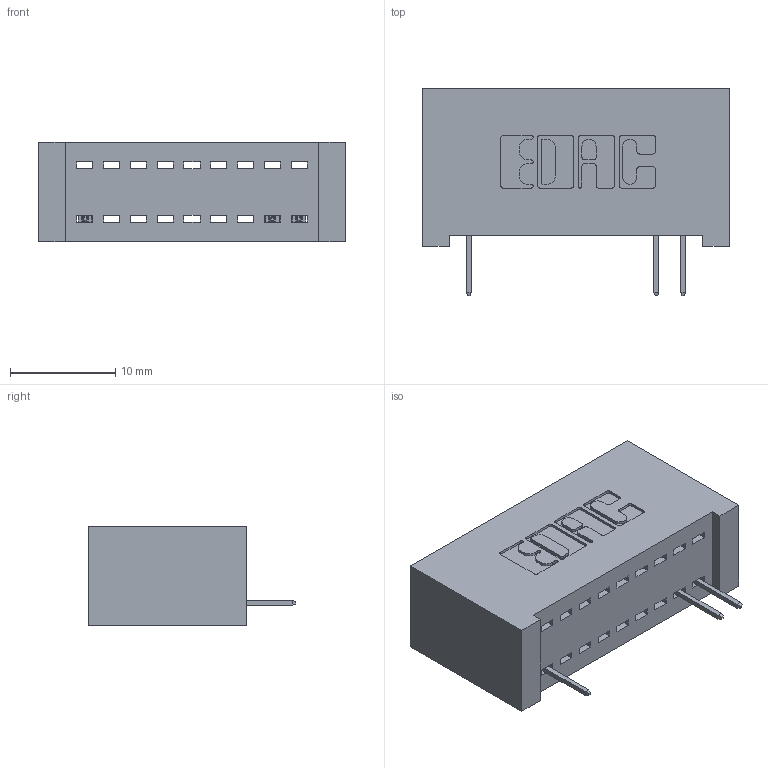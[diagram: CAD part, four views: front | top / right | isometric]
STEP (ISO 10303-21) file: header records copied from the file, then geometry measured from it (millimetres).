
FILE_DESCRIPTION (( 'STEP AP203' ), '1' );
FILE_NAME ('392-009-524-101.STEP', '2018-08-14T19:42:58', ( '' ), ( '' ), 'SwSTEP 2.0', 'SolidWorks 2016', '' );
FILE_SCHEMA (( 'CONFIG_CONTROL_DESIGN' ));
Length unit declared in the file: inch
Products named in the file (3): 345-292-001_345-293-124; 392-009-524-101; 342 Part_Lugless
Assembly tree (4 placements, depth 2):
  392-009-524-101
    342 Part_Lugless
    345-292-001_345-293-124  x3
Bounding box: 29.11 x 19.69 x 9.4 mm (x, y, z)
Volume: 2759.2 mm3; surface area: 3366.5 mm2
Topology: 4 solids, 4 shells, 360 faces, 1067 edges, 698 vertices
Faces by surface type: plane 278, cylinder 82
Entity records: 9243 total; most frequent: CARTESIAN_POINT 1631, ORIENTED_EDGE 1582, DIRECTION 1429, EDGE_CURVE 791, VECTOR 675, LINE 675, VERTEX_POINT 522, AXIS2_PLACEMENT_3D 377
